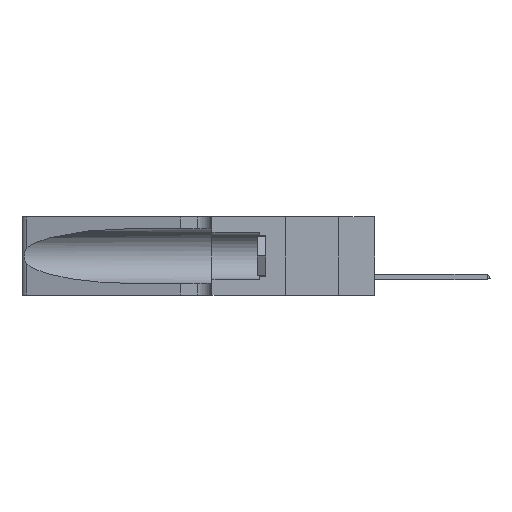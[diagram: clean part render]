
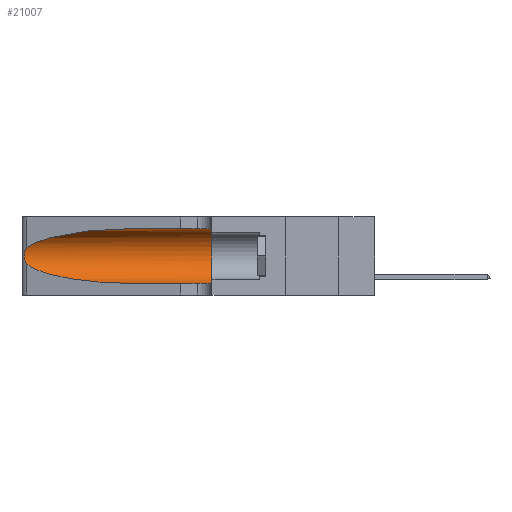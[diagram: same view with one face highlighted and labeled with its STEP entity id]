
A CAD part, left-side view. The second image highlights one B-rep face of the part: STEP entity #21007.
In plain terms, the highlighted cylindrical face has radius 3.308 mm (diameter 6.617 mm), a partial arc.
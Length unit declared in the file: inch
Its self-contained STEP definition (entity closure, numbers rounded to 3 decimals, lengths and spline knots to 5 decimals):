
#10 = B_SPLINE_CURVE_WITH_KNOTS ( 'NONE', 3,
 ( #11604, #8752, #23081, #20260, #32330, #2536, #5524, #5890, #20833, #24137, #35553, #20943, #23905, #26886 ),
 .UNSPECIFIED., .F., .F.,
 ( 4, 2, 2, 2, 2, 2, 4 ),
 ( 0., 0.00027, 0.00053, 0.00107, 0.0016, 0.00187, 0.00214 ),
 .UNSPECIFIED. ) ;
#2536 = CARTESIAN_POINT ( 'NONE',  ( 0.26018, 1.23835, 0.19895 ) ) ;
#3510 = CARTESIAN_POINT ( 'NONE',  ( 0.1305, 0.35, 0.05475 ) ) ;
#3540 = DIRECTION ( 'NONE',  ( 0., 0., -1. ) ) ;
#4692 = CARTESIAN_POINT ( 'NONE',  ( 0.1305, 0.35, 0.185 ) ) ;
#5375 = VERTEX_POINT ( 'NONE', #24996 ) ;
#5524 = CARTESIAN_POINT ( 'NONE',  ( 0.26075, 1.23896, 0.19203 ) ) ;
#5672 = CARTESIAN_POINT ( 'NONE',  ( 0.25487, 1.22718, 0.22369 ) ) ;
#5890 = CARTESIAN_POINT ( 'NONE',  ( 0.26075, 1.23896, 0.178 ) ) ;
#7273 = DIRECTION ( 'NONE',  ( 0., 0., 1. ) ) ;
#7387 = ORIENTED_EDGE ( 'NONE', *, *, #17015, .F. ) ;
#8633 = AXIS2_PLACEMENT_3D ( 'NONE', #32614, #30001, #3540 ) ;
#8752 = CARTESIAN_POINT ( 'NONE',  ( 0.25555, 1.22994, 0.2215 ) ) ;
#8874 = CARTESIAN_POINT ( 'NONE',  ( 0.18966, 0.96281, 0.31525 ) ) ;
#9155 = VECTOR ( 'NONE', #11594, 39.37008 ) ;
#9242 = VERTEX_POINT ( 'NONE', #19439 ) ;
#10120 = CARTESIAN_POINT ( 'NONE',  ( 0.25487, 1.22718, 0.14631 ) ) ;
#10386 = DIRECTION ( 'NONE',  ( 0., 1., 0. ) ) ;
#11594 = DIRECTION ( 'NONE',  ( 0., -1., 0. ) ) ;
#11604 = CARTESIAN_POINT ( 'NONE',  ( 0.25487, 1.22718, 0.22369 ) ) ;
#11995 = VERTEX_POINT ( 'NONE', #10120 ) ;
#12964 = CARTESIAN_POINT ( 'NONE',  ( 0.25487, 1.22718, 0.14631 ) ) ;
#13841 = CARTESIAN_POINT ( 'NONE',  ( 0.1305, 0.35, 0.31525 ) ) ;
#14924 =( BOUNDED_CURVE ( )  B_SPLINE_CURVE ( 3, ( #12964, #33961, #25056, #27634 ),
 .UNSPECIFIED., .F., .F. ) 
 B_SPLINE_CURVE_WITH_KNOTS ( ( 4, 4 ),
 ( 3.44316, 4.71239 ),
 .UNSPECIFIED. ) 
 CURVE ( )  GEOMETRIC_REPRESENTATION_ITEM ( )  RATIONAL_B_SPLINE_CURVE ( ( 1., 0.87, 0.87, 1. ) ) 
 REPRESENTATION_ITEM ( '' )  );
#17015 = EDGE_CURVE ( 'NONE', #18695, #18026, #23476, .T. ) ;
#17045 = DIRECTION ( 'NONE',  ( 0., -1., 0. ) ) ;
#17662 = CARTESIAN_POINT ( 'NONE',  ( 0.1305, 0.72297, 0.31525 ) ) ;
#18026 = VERTEX_POINT ( 'NONE', #3510 ) ;
#18385 = EDGE_CURVE ( 'NONE', #5375, #11995, #10, .T. ) ;
#18488 = CARTESIAN_POINT ( 'NONE',  ( 0.1305, 0.72297, 0.05475 ) ) ;
#18695 = VERTEX_POINT ( 'NONE', #13841 ) ;
#19120 = FACE_OUTER_BOUND ( 'NONE', #20759, .T. ) ;
#19296 = ORIENTED_EDGE ( 'NONE', *, *, #24117, .T. ) ;
#19439 = CARTESIAN_POINT ( 'NONE',  ( 0.1305, 0.72297, 0.31525 ) ) ;
#19531 = VERTEX_POINT ( 'NONE', #18488 ) ;
#20139 = CARTESIAN_POINT ( 'NONE',  ( 0.1305, 1.61858, 0.31525 ) ) ;
#20260 = CARTESIAN_POINT ( 'NONE',  ( 0.25787, 1.23484, 0.2124 ) ) ;
#20759 = EDGE_LOOP ( 'NONE', ( #27678, #24770, #27263, #19296, #7387, #23565 ) ) ;
#20833 = CARTESIAN_POINT ( 'NONE',  ( 0.26017, 1.23833, 0.17102 ) ) ;
#20943 = CARTESIAN_POINT ( 'NONE',  ( 0.25639, 1.23186, 0.15144 ) ) ;
#21007 = ADVANCED_FACE ( 'NONE', ( #19120 ), #34354, .F. ) ;
#21070 = EDGE_CURVE ( 'NONE', #9242, #5375, #22278, .T. ) ;
#22278 =( BOUNDED_CURVE ( )  B_SPLINE_CURVE ( 3, ( #17662, #8874, #23336, #5672 ),
 .UNSPECIFIED., .F., .T. ) 
 B_SPLINE_CURVE_WITH_KNOTS ( ( 4, 4 ),
 ( 1.5708, 2.84003 ),
 .UNSPECIFIED. ) 
 CURVE ( )  GEOMETRIC_REPRESENTATION_ITEM ( )  RATIONAL_B_SPLINE_CURVE ( ( 1., 0.87, 0.87, 1. ) ) 
 REPRESENTATION_ITEM ( '' )  );
#23081 = CARTESIAN_POINT ( 'NONE',  ( 0.25639, 1.23184, 0.21858 ) ) ;
#23336 = CARTESIAN_POINT ( 'NONE',  ( 0.2373, 1.15595, 0.28018 ) ) ;
#23476 = CIRCLE ( 'NONE', #33281, 0.13025 ) ;
#23565 = ORIENTED_EDGE ( 'NONE', *, *, #35828, .F. ) ;
#23905 = CARTESIAN_POINT ( 'NONE',  ( 0.25555, 1.22993, 0.14849 ) ) ;
#24117 = EDGE_CURVE ( 'NONE', #19531, #18026, #32288, .T. ) ;
#24137 = CARTESIAN_POINT ( 'NONE',  ( 0.25856, 1.23593, 0.16098 ) ) ;
#24770 = ORIENTED_EDGE ( 'NONE', *, *, #18385, .T. ) ;
#24996 = CARTESIAN_POINT ( 'NONE',  ( 0.25487, 1.22718, 0.22369 ) ) ;
#25056 = CARTESIAN_POINT ( 'NONE',  ( 0.18966, 0.96281, 0.05475 ) ) ;
#26037 = CARTESIAN_POINT ( 'NONE',  ( 0.1305, 1.61858, 0.05475 ) ) ;
#26886 = CARTESIAN_POINT ( 'NONE',  ( 0.25487, 1.22718, 0.14631 ) ) ;
#27263 = ORIENTED_EDGE ( 'NONE', *, *, #31813, .T. ) ;
#27634 = CARTESIAN_POINT ( 'NONE',  ( 0.1305, 0.72297, 0.05475 ) ) ;
#27678 = ORIENTED_EDGE ( 'NONE', *, *, #21070, .T. ) ;
#30001 = DIRECTION ( 'NONE',  ( 0., -1., 0. ) ) ;
#31813 = EDGE_CURVE ( 'NONE', #11995, #19531, #14924, .T. ) ;
#32288 = LINE ( 'NONE', #26037, #9155 ) ;
#32330 = CARTESIAN_POINT ( 'NONE',  ( 0.25854, 1.2359, 0.20912 ) ) ;
#32614 = CARTESIAN_POINT ( 'NONE',  ( 0.1305, 1.61858, 0.185 ) ) ;
#33281 = AXIS2_PLACEMENT_3D ( 'NONE', #4692, #10386, #7273 ) ;
#33961 = CARTESIAN_POINT ( 'NONE',  ( 0.2373, 1.15595, 0.08982 ) ) ;
#34354 = CYLINDRICAL_SURFACE ( 'NONE', #8633, 0.13025 ) ;
#34424 = LINE ( 'NONE', #20139, #35751 ) ;
#35553 = CARTESIAN_POINT ( 'NONE',  ( 0.25789, 1.23486, 0.15765 ) ) ;
#35751 = VECTOR ( 'NONE', #17045, 39.37008 ) ;
#35828 = EDGE_CURVE ( 'NONE', #9242, #18695, #34424, .T. ) ;
